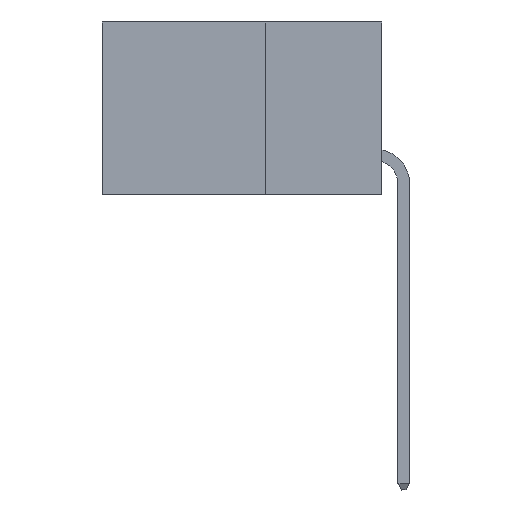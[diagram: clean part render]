
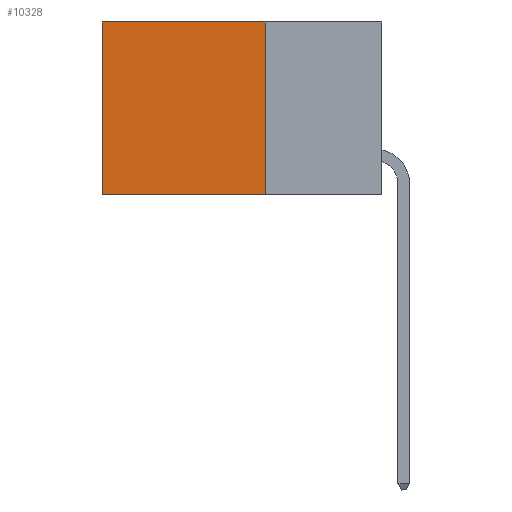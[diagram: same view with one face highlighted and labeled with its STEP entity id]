
A CAD part, left-side view. The second image highlights one B-rep face of the part: STEP entity #10328.
In plain terms, the highlighted planar face has unit normal (-1, 0, 0).
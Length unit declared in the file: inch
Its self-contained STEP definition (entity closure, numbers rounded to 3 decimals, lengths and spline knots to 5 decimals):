
#708 = EDGE_LOOP ( 'NONE', ( #8772, #1622, #14253, #15407 ) ) ;
#1510 = LINE ( 'NONE', #7914, #16361 ) ;
#1622 = ORIENTED_EDGE ( 'NONE', *, *, #8193, .F. ) ;
#2585 = PLANE ( 'NONE',  #4365 ) ;
#2734 = VECTOR ( 'NONE', #5512, 39.37008 ) ;
#2780 = CARTESIAN_POINT ( 'NONE',  ( 0.2875, 0.25, 0. ) ) ;
#3889 = CARTESIAN_POINT ( 'NONE',  ( 0.2875, 0.25, 0. ) ) ;
#4365 = AXIS2_PLACEMENT_3D ( 'NONE', #11208, #8505, #5636 ) ;
#5288 = EDGE_CURVE ( 'NONE', #14199, #9390, #14732, .T. ) ;
#5512 = DIRECTION ( 'NONE',  ( 0., 1., 0. ) ) ;
#5636 = DIRECTION ( 'NONE',  ( 0., 0., -1. ) ) ;
#6747 = CARTESIAN_POINT ( 'NONE',  ( 0.2875, 0.25, -0.37 ) ) ;
#7413 = VECTOR ( 'NONE', #10650, 39.37008 ) ;
#7914 = CARTESIAN_POINT ( 'NONE',  ( 0.2875, 0.25, 0. ) ) ;
#8082 = FACE_OUTER_BOUND ( 'NONE', #708, .T. ) ;
#8193 = EDGE_CURVE ( 'NONE', #11632, #16192, #10196, .T. ) ;
#8505 = DIRECTION ( 'NONE',  ( 1., 0., 0. ) ) ;
#8772 = ORIENTED_EDGE ( 'NONE', *, *, #9020, .T. ) ;
#9020 = EDGE_CURVE ( 'NONE', #9390, #16192, #13955, .T. ) ;
#9390 = VERTEX_POINT ( 'NONE', #11981 ) ;
#10196 = LINE ( 'NONE', #6747, #2734 ) ;
#10328 = ADVANCED_FACE ( 'NONE', ( #8082 ), #2585, .F. ) ;
#10650 = DIRECTION ( 'NONE',  ( 0., 0., -1. ) ) ;
#11208 = CARTESIAN_POINT ( 'NONE',  ( 0.2875, 0.25, 0. ) ) ;
#11632 = VERTEX_POINT ( 'NONE', #16836 ) ;
#11981 = CARTESIAN_POINT ( 'NONE',  ( 0.2875, 0.6, 0. ) ) ;
#13955 = LINE ( 'NONE', #15139, #7413 ) ;
#14199 = VERTEX_POINT ( 'NONE', #2780 ) ;
#14253 = ORIENTED_EDGE ( 'NONE', *, *, #17323, .F. ) ;
#14732 = LINE ( 'NONE', #3889, #16734 ) ;
#15139 = CARTESIAN_POINT ( 'NONE',  ( 0.2875, 0.6, 0. ) ) ;
#15144 = DIRECTION ( 'NONE',  ( 0., 1., 0. ) ) ;
#15407 = ORIENTED_EDGE ( 'NONE', *, *, #5288, .T. ) ;
#16192 = VERTEX_POINT ( 'NONE', #16347 ) ;
#16347 = CARTESIAN_POINT ( 'NONE',  ( 0.2875, 0.6, -0.37 ) ) ;
#16361 = VECTOR ( 'NONE', #17977, 39.37008 ) ;
#16734 = VECTOR ( 'NONE', #15144, 39.37008 ) ;
#16836 = CARTESIAN_POINT ( 'NONE',  ( 0.2875, 0.25, -0.37 ) ) ;
#17323 = EDGE_CURVE ( 'NONE', #14199, #11632, #1510, .T. ) ;
#17977 = DIRECTION ( 'NONE',  ( 0., 0., -1. ) ) ;
